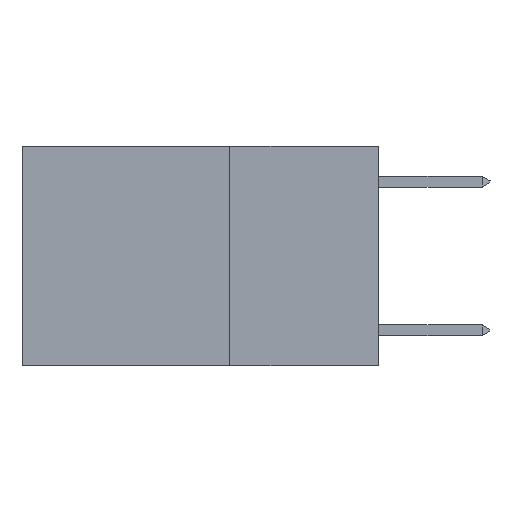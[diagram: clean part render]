
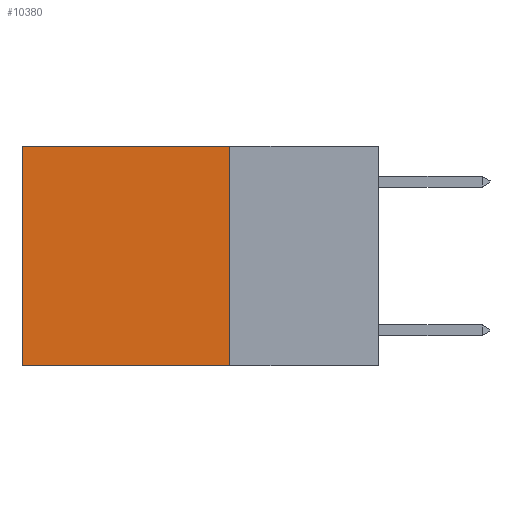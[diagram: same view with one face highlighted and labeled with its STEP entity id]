
A CAD part, left-side view. The second image highlights one B-rep face of the part: STEP entity #10380.
In plain terms, the highlighted planar face has unit normal (-1, 0, 0).
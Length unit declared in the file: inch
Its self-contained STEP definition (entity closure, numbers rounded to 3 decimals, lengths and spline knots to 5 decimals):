
#697 = ORIENTED_EDGE ( 'NONE', *, *, #5588, .T. ) ;
#1161 = VECTOR ( 'NONE', #6695, 39.37008 ) ;
#1605 = CARTESIAN_POINT ( 'NONE',  ( 0.2625, 0.25, 0. ) ) ;
#2045 = CARTESIAN_POINT ( 'NONE',  ( 0.2625, 0.6, 0. ) ) ;
#2709 = CARTESIAN_POINT ( 'NONE',  ( 0.2625, 0.25, -0.37 ) ) ;
#2813 = DIRECTION ( 'NONE',  ( 0., 0., -1. ) ) ;
#2991 = ORIENTED_EDGE ( 'NONE', *, *, #3076, .F. ) ;
#3076 = EDGE_CURVE ( 'NONE', #7301, #7318, #10360, .T. ) ;
#3341 = LINE ( 'NONE', #2709, #1161 ) ;
#4298 = CARTESIAN_POINT ( 'NONE',  ( 0.2625, 0.25, 0. ) ) ;
#4344 = DIRECTION ( 'NONE',  ( 0., 0., -1. ) ) ;
#4434 = ORIENTED_EDGE ( 'NONE', *, *, #4511, .T. ) ;
#4511 = EDGE_CURVE ( 'NONE', #7609, #8725, #5610, .T. ) ;
#4698 = CARTESIAN_POINT ( 'NONE',  ( 0.2625, 0.25, -0.37 ) ) ;
#5215 = PLANE ( 'NONE',  #8502 ) ;
#5588 = EDGE_CURVE ( 'NONE', #7301, #7609, #8314, .T. ) ;
#5610 = LINE ( 'NONE', #7470, #9593 ) ;
#6361 = VECTOR ( 'NONE', #9026, 39.37008 ) ;
#6695 = DIRECTION ( 'NONE',  ( 0., 1., 0. ) ) ;
#7242 = CARTESIAN_POINT ( 'NONE',  ( 0.2625, 0.25, 0. ) ) ;
#7301 = VERTEX_POINT ( 'NONE', #7242 ) ;
#7318 = VERTEX_POINT ( 'NONE', #4698 ) ;
#7470 = CARTESIAN_POINT ( 'NONE',  ( 0.2625, 0.6, 0. ) ) ;
#7559 = CARTESIAN_POINT ( 'NONE',  ( 0.2625, 0.25, 0. ) ) ;
#7596 = DIRECTION ( 'NONE',  ( 1., 0., 0. ) ) ;
#7609 = VERTEX_POINT ( 'NONE', #2045 ) ;
#7845 = EDGE_LOOP ( 'NONE', ( #4434, #9464, #2991, #697 ) ) ;
#8314 = LINE ( 'NONE', #1605, #10195 ) ;
#8502 = AXIS2_PLACEMENT_3D ( 'NONE', #7559, #7596, #2813 ) ;
#8725 = VERTEX_POINT ( 'NONE', #8975 ) ;
#8797 = DIRECTION ( 'NONE',  ( 0., 1., 0. ) ) ;
#8975 = CARTESIAN_POINT ( 'NONE',  ( 0.2625, 0.6, -0.37 ) ) ;
#9026 = DIRECTION ( 'NONE',  ( 0., 0., -1. ) ) ;
#9201 = FACE_OUTER_BOUND ( 'NONE', #7845, .T. ) ;
#9464 = ORIENTED_EDGE ( 'NONE', *, *, #10307, .F. ) ;
#9593 = VECTOR ( 'NONE', #4344, 39.37008 ) ;
#10195 = VECTOR ( 'NONE', #8797, 39.37008 ) ;
#10307 = EDGE_CURVE ( 'NONE', #7318, #8725, #3341, .T. ) ;
#10360 = LINE ( 'NONE', #4298, #6361 ) ;
#10380 = ADVANCED_FACE ( 'NONE', ( #9201 ), #5215, .F. ) ;
